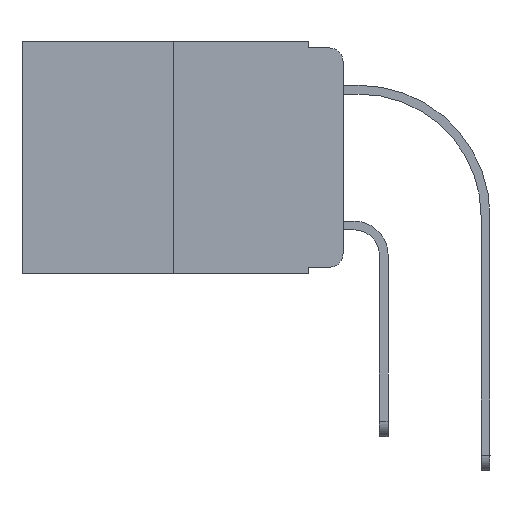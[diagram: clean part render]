
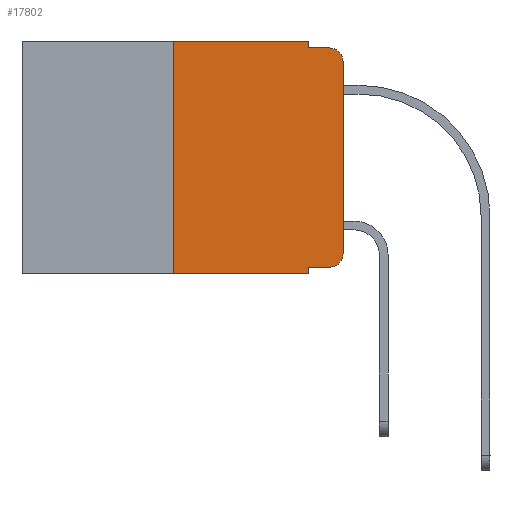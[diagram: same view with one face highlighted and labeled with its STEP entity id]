
A CAD part, left-side view. The second image highlights one B-rep face of the part: STEP entity #17802.
In plain terms, the highlighted planar face has unit normal (-1, 0, 0).
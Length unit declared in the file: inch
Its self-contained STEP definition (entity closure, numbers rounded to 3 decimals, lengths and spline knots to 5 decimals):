
#171 = LINE ( 'NONE', #16006, #3672 ) ;
#295 = CARTESIAN_POINT ( 'NONE',  ( 0., 0.02, -0.03 ) ) ;
#335 = CARTESIAN_POINT ( 'NONE',  ( 0., 0.051, -0.01 ) ) ;
#614 = CARTESIAN_POINT ( 'NONE',  ( 0., 0.473, 0. ) ) ;
#691 = VECTOR ( 'NONE', #6805, 39.37008 ) ;
#930 = AXIS2_PLACEMENT_3D ( 'NONE', #2928, #16911, #7597 ) ;
#1311 = DIRECTION ( 'NONE',  ( 0., 0., -1. ) ) ;
#1385 = EDGE_CURVE ( 'NONE', #17877, #5760, #7586, .T. ) ;
#1460 = ORIENTED_EDGE ( 'NONE', *, *, #4322, .T. ) ;
#1856 = DIRECTION ( 'NONE',  ( 0., -1., 0. ) ) ;
#1968 = EDGE_CURVE ( 'NONE', #2644, #18191, #18767, .T. ) ;
#2218 = VECTOR ( 'NONE', #14714, 39.37008 ) ;
#2583 = CARTESIAN_POINT ( 'NONE',  ( 0., 0.25, 0. ) ) ;
#2644 = VERTEX_POINT ( 'NONE', #5399 ) ;
#2864 = DIRECTION ( 'NONE',  ( 1., 0., 0. ) ) ;
#2893 = LINE ( 'NONE', #10861, #17720 ) ;
#2928 = CARTESIAN_POINT ( 'NONE',  ( 0., 0.02, -0.313 ) ) ;
#2954 = AXIS2_PLACEMENT_3D ( 'NONE', #295, #13034, #11373 ) ;
#3084 = ORIENTED_EDGE ( 'NONE', *, *, #9309, .F. ) ;
#3672 = VECTOR ( 'NONE', #8146, 39.37008 ) ;
#4322 = EDGE_CURVE ( 'NONE', #6025, #5308, #11372, .T. ) ;
#4372 = DIRECTION ( 'NONE',  ( 0., 0., 1. ) ) ;
#4478 = ORIENTED_EDGE ( 'NONE', *, *, #1385, .T. ) ;
#4660 = VECTOR ( 'NONE', #20168, 39.37008 ) ;
#4760 = ORIENTED_EDGE ( 'NONE', *, *, #6949, .F. ) ;
#4784 = CARTESIAN_POINT ( 'NONE',  ( 0., 0.051, 0. ) ) ;
#4880 = ORIENTED_EDGE ( 'NONE', *, *, #17286, .F. ) ;
#5308 = VERTEX_POINT ( 'NONE', #10267 ) ;
#5399 = CARTESIAN_POINT ( 'NONE',  ( 0., 0.02, -0.333 ) ) ;
#5699 = CARTESIAN_POINT ( 'NONE',  ( 0., 0.02, -0.01 ) ) ;
#5760 = VERTEX_POINT ( 'NONE', #5699 ) ;
#6025 = VERTEX_POINT ( 'NONE', #17874 ) ;
#6066 = EDGE_CURVE ( 'NONE', #6835, #2644, #11555, .T. ) ;
#6086 = EDGE_CURVE ( 'NONE', #6835, #5308, #171, .T. ) ;
#6732 = DIRECTION ( 'NONE',  ( 0., -1., 0. ) ) ;
#6805 = DIRECTION ( 'NONE',  ( 0., -1., 0. ) ) ;
#6813 = VECTOR ( 'NONE', #12439, 39.37008 ) ;
#6835 = VERTEX_POINT ( 'NONE', #7598 ) ;
#6949 = EDGE_CURVE ( 'NONE', #8890, #8729, #14587, .T. ) ;
#7586 = CIRCLE ( 'NONE', #2954, 0.02 ) ;
#7597 = DIRECTION ( 'NONE',  ( 0., 0., -1. ) ) ;
#7598 = CARTESIAN_POINT ( 'NONE',  ( 0., 0.051, -0.333 ) ) ;
#8146 = DIRECTION ( 'NONE',  ( 0., 0., -1. ) ) ;
#8658 = VECTOR ( 'NONE', #1856, 39.37008 ) ;
#8729 = VERTEX_POINT ( 'NONE', #17423 ) ;
#8890 = VERTEX_POINT ( 'NONE', #14948 ) ;
#9309 = EDGE_CURVE ( 'NONE', #13001, #5760, #11623, .T. ) ;
#9945 = ORIENTED_EDGE ( 'NONE', *, *, #1968, .T. ) ;
#10267 = CARTESIAN_POINT ( 'NONE',  ( 0., 0.051, -0.343 ) ) ;
#10483 = CARTESIAN_POINT ( 'NONE',  ( 0., 0.051, -0.01 ) ) ;
#10738 = CARTESIAN_POINT ( 'NONE',  ( 0., 0.473, 0. ) ) ;
#10861 = CARTESIAN_POINT ( 'NONE',  ( 0., 0., 0. ) ) ;
#11353 = CARTESIAN_POINT ( 'NONE',  ( 0., 0.051, -0.333 ) ) ;
#11372 = LINE ( 'NONE', #14683, #8658 ) ;
#11373 = DIRECTION ( 'NONE',  ( 0., 0., -1. ) ) ;
#11555 = LINE ( 'NONE', #11353, #691 ) ;
#11623 = LINE ( 'NONE', #335, #2218 ) ;
#12439 = DIRECTION ( 'NONE',  ( 0., 0., -1. ) ) ;
#12772 = ORIENTED_EDGE ( 'NONE', *, *, #6066, .T. ) ;
#13001 = VERTEX_POINT ( 'NONE', #10483 ) ;
#13034 = DIRECTION ( 'NONE',  ( -1., 0., 0. ) ) ;
#13130 = EDGE_CURVE ( 'NONE', #8729, #13001, #14296, .T. ) ;
#13597 = EDGE_CURVE ( 'NONE', #18191, #17877, #2893, .T. ) ;
#14296 = LINE ( 'NONE', #4784, #6813 ) ;
#14587 = LINE ( 'NONE', #614, #19248 ) ;
#14683 = CARTESIAN_POINT ( 'NONE',  ( 0., 0.473, -0.343 ) ) ;
#14714 = DIRECTION ( 'NONE',  ( 0., -1., 0. ) ) ;
#14948 = CARTESIAN_POINT ( 'NONE',  ( 0., 0.25, 0. ) ) ;
#16006 = CARTESIAN_POINT ( 'NONE',  ( 0., 0.051, 0. ) ) ;
#16122 = ORIENTED_EDGE ( 'NONE', *, *, #6086, .F. ) ;
#16573 = AXIS2_PLACEMENT_3D ( 'NONE', #10738, #2864, #1311 ) ;
#16911 = DIRECTION ( 'NONE',  ( -1., 0., 0. ) ) ;
#17038 = FACE_OUTER_BOUND ( 'NONE', #17467, .T. ) ;
#17286 = EDGE_CURVE ( 'NONE', #6025, #8890, #20059, .T. ) ;
#17423 = CARTESIAN_POINT ( 'NONE',  ( 0., 0.051, 0. ) ) ;
#17467 = EDGE_LOOP ( 'NONE', ( #20256, #4478, #3084, #20061, #4760, #4880, #1460, #16122, #12772, #9945 ) ) ;
#17720 = VECTOR ( 'NONE', #4372, 39.37008 ) ;
#17802 = ADVANCED_FACE ( 'NONE', ( #17038 ), #18693, .F. ) ;
#17874 = CARTESIAN_POINT ( 'NONE',  ( 0., 0.25, -0.343 ) ) ;
#17877 = VERTEX_POINT ( 'NONE', #18895 ) ;
#18191 = VERTEX_POINT ( 'NONE', #20115 ) ;
#18693 = PLANE ( 'NONE',  #16573 ) ;
#18767 = CIRCLE ( 'NONE', #930, 0.02 ) ;
#18895 = CARTESIAN_POINT ( 'NONE',  ( 0., 0., -0.03 ) ) ;
#19248 = VECTOR ( 'NONE', #6732, 39.37008 ) ;
#20059 = LINE ( 'NONE', #2583, #4660 ) ;
#20061 = ORIENTED_EDGE ( 'NONE', *, *, #13130, .F. ) ;
#20115 = CARTESIAN_POINT ( 'NONE',  ( 0., 0., -0.313 ) ) ;
#20168 = DIRECTION ( 'NONE',  ( 0., 0., 1. ) ) ;
#20256 = ORIENTED_EDGE ( 'NONE', *, *, #13597, .T. ) ;
